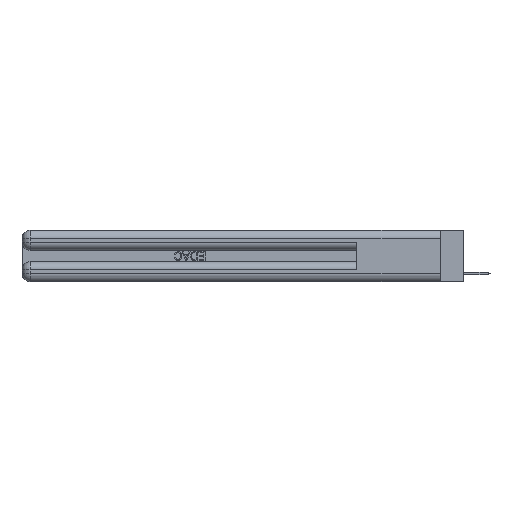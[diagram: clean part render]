
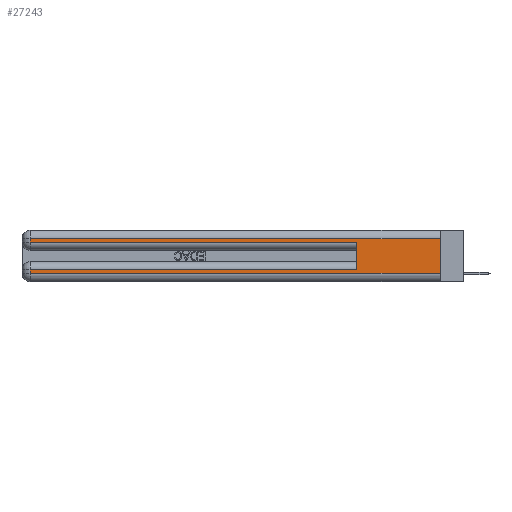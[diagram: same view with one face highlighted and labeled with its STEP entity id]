
A CAD part, left-side view. The second image highlights one B-rep face of the part: STEP entity #27243.
In plain terms, the highlighted planar face has unit normal (-1, 0, 0).
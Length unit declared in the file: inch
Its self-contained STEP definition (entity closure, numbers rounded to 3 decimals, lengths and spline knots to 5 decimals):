
#88 = CARTESIAN_POINT ( 'NONE',  ( 0., 2.94, 0.31 ) ) ;
#712 = VECTOR ( 'NONE', #2915, 39.37008 ) ;
#754 = ORIENTED_EDGE ( 'NONE', *, *, #22117, .T. ) ;
#1409 = VECTOR ( 'NONE', #28734, 39.37008 ) ;
#1683 = ORIENTED_EDGE ( 'NONE', *, *, #27415, .T. ) ;
#1808 = VERTEX_POINT ( 'NONE', #28199 ) ;
#2278 = DIRECTION ( 'NONE',  ( 1., 0., 0. ) ) ;
#2288 = CARTESIAN_POINT ( 'NONE',  ( 0., 2.94, 0.37 ) ) ;
#2559 = ORIENTED_EDGE ( 'NONE', *, *, #27789, .T. ) ;
#2640 = EDGE_CURVE ( 'NONE', #12469, #29110, #29205, .T. ) ;
#2915 = DIRECTION ( 'NONE',  ( 0., 1., 0. ) ) ;
#3526 = CARTESIAN_POINT ( 'NONE',  ( 0., 0., 0.31 ) ) ;
#4398 = DIRECTION ( 'NONE',  ( 0., 0., -1. ) ) ;
#4934 = VECTOR ( 'NONE', #7638, 39.37008 ) ;
#5937 = EDGE_CURVE ( 'NONE', #24942, #31499, #22830, .T. ) ;
#6096 = DIRECTION ( 'NONE',  ( 0., -1., 0. ) ) ;
#6153 = DIRECTION ( 'NONE',  ( 0., 1., 0. ) ) ;
#7427 = CARTESIAN_POINT ( 'NONE',  ( 0., 2.94, 0.37 ) ) ;
#7454 = EDGE_CURVE ( 'NONE', #12469, #19887, #16698, .T. ) ;
#7638 = DIRECTION ( 'NONE',  ( 0., -1., 0. ) ) ;
#8853 = CARTESIAN_POINT ( 'NONE',  ( 0., 0., 0.285 ) ) ;
#9246 = PLANE ( 'NONE',  #16389 ) ;
#11485 = VECTOR ( 'NONE', #6096, 39.37008 ) ;
#12469 = VERTEX_POINT ( 'NONE', #23209 ) ;
#13409 = VERTEX_POINT ( 'NONE', #31139 ) ;
#14163 = EDGE_LOOP ( 'NONE', ( #22632, #17559, #29238, #1683, #27741, #22906, #2559, #754 ) ) ;
#14651 = LINE ( 'NONE', #7427, #30602 ) ;
#15063 = CARTESIAN_POINT ( 'NONE',  ( 0., 0., 0.085 ) ) ;
#16389 = AXIS2_PLACEMENT_3D ( 'NONE', #31388, #2278, #30950 ) ;
#16698 = LINE ( 'NONE', #23782, #1409 ) ;
#17199 = VERTEX_POINT ( 'NONE', #27034 ) ;
#17499 = DIRECTION ( 'NONE',  ( 0., 0., -1. ) ) ;
#17559 = ORIENTED_EDGE ( 'NONE', *, *, #5937, .T. ) ;
#18037 = LINE ( 'NONE', #8853, #11485 ) ;
#19304 = EDGE_CURVE ( 'NONE', #31499, #17199, #14651, .T. ) ;
#19874 = LINE ( 'NONE', #22179, #4934 ) ;
#19887 = VERTEX_POINT ( 'NONE', #29058 ) ;
#19910 = LINE ( 'NONE', #2288, #26681 ) ;
#21519 = CARTESIAN_POINT ( 'NONE',  ( 0., 0., 0.37 ) ) ;
#22117 = EDGE_CURVE ( 'NONE', #13409, #1808, #19874, .T. ) ;
#22179 = CARTESIAN_POINT ( 'NONE',  ( 0., 0., 0.06 ) ) ;
#22632 = ORIENTED_EDGE ( 'NONE', *, *, #24781, .F. ) ;
#22830 = LINE ( 'NONE', #3526, #24304 ) ;
#22906 = ORIENTED_EDGE ( 'NONE', *, *, #2640, .T. ) ;
#22966 = FACE_OUTER_BOUND ( 'NONE', #14163, .T. ) ;
#23209 = CARTESIAN_POINT ( 'NONE',  ( 0., 0.6, 0.085 ) ) ;
#23782 = CARTESIAN_POINT ( 'NONE',  ( 0., 0.6, 0.145 ) ) ;
#24109 = DIRECTION ( 'NONE',  ( 0., 0., -1. ) ) ;
#24304 = VECTOR ( 'NONE', #6153, 39.37008 ) ;
#24781 = EDGE_CURVE ( 'NONE', #24942, #1808, #28752, .T. ) ;
#24942 = VERTEX_POINT ( 'NONE', #26851 ) ;
#25723 = VECTOR ( 'NONE', #24109, 39.37008 ) ;
#26681 = VECTOR ( 'NONE', #4398, 39.37008 ) ;
#26851 = CARTESIAN_POINT ( 'NONE',  ( 0., 0., 0.31 ) ) ;
#27034 = CARTESIAN_POINT ( 'NONE',  ( 0., 2.94, 0.285 ) ) ;
#27243 = ADVANCED_FACE ( 'NONE', ( #22966 ), #9246, .F. ) ;
#27415 = EDGE_CURVE ( 'NONE', #17199, #19887, #18037, .T. ) ;
#27741 = ORIENTED_EDGE ( 'NONE', *, *, #7454, .F. ) ;
#27789 = EDGE_CURVE ( 'NONE', #29110, #13409, #19910, .T. ) ;
#28199 = CARTESIAN_POINT ( 'NONE',  ( 0., 0., 0.06 ) ) ;
#28734 = DIRECTION ( 'NONE',  ( 0., 0., 1. ) ) ;
#28752 = LINE ( 'NONE', #21519, #25723 ) ;
#28939 = CARTESIAN_POINT ( 'NONE',  ( 0., 2.94, 0.085 ) ) ;
#29058 = CARTESIAN_POINT ( 'NONE',  ( 0., 0.6, 0.285 ) ) ;
#29110 = VERTEX_POINT ( 'NONE', #28939 ) ;
#29205 = LINE ( 'NONE', #15063, #712 ) ;
#29238 = ORIENTED_EDGE ( 'NONE', *, *, #19304, .T. ) ;
#30602 = VECTOR ( 'NONE', #17499, 39.37008 ) ;
#30950 = DIRECTION ( 'NONE',  ( 0., 0., -1. ) ) ;
#31139 = CARTESIAN_POINT ( 'NONE',  ( 0., 2.94, 0.06 ) ) ;
#31388 = CARTESIAN_POINT ( 'NONE',  ( 0., 0., 0.37 ) ) ;
#31499 = VERTEX_POINT ( 'NONE', #88 ) ;
